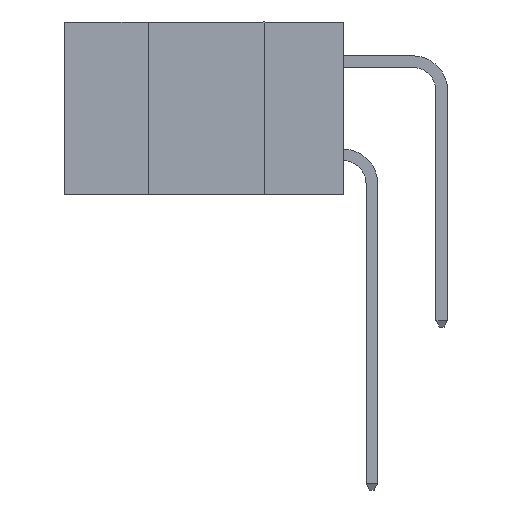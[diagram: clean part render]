
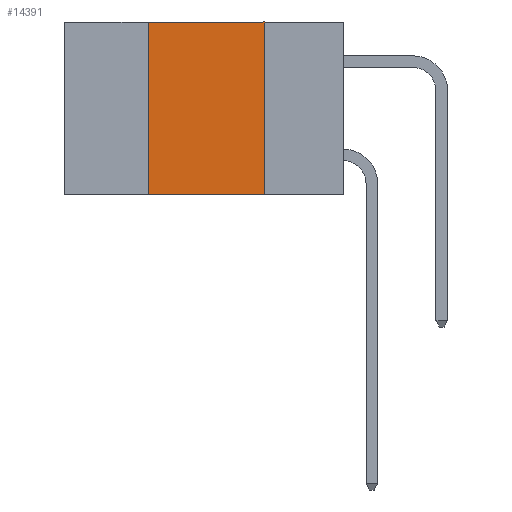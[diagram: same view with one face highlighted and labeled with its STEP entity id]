
A CAD part, left-side view. The second image highlights one B-rep face of the part: STEP entity #14391.
In plain terms, the highlighted planar face has unit normal (-1, 0, 0).
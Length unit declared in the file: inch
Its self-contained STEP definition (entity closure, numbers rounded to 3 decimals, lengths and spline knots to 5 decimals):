
#1706 = LINE ( 'NONE', #13991, #2848 ) ;
#2848 = VECTOR ( 'NONE', #13791, 39.37008 ) ;
#4884 = PLANE ( 'NONE',  #15498 ) ;
#5731 = VERTEX_POINT ( 'NONE', #10891 ) ;
#5781 = LINE ( 'NONE', #11690, #9344 ) ;
#6665 = DIRECTION ( 'NONE',  ( 0., 0., -1. ) ) ;
#6890 = CARTESIAN_POINT ( 'NONE',  ( 0., 0.17, -0.37 ) ) ;
#6941 = ORIENTED_EDGE ( 'NONE', *, *, #12278, .F. ) ;
#7290 = EDGE_LOOP ( 'NONE', ( #6941, #21047, #7484, #17150 ) ) ;
#7484 = ORIENTED_EDGE ( 'NONE', *, *, #7670, .F. ) ;
#7536 = CARTESIAN_POINT ( 'NONE',  ( 0., 0.42, 0. ) ) ;
#7670 = EDGE_CURVE ( 'NONE', #5731, #15430, #1706, .T. ) ;
#9344 = VECTOR ( 'NONE', #16772, 39.37008 ) ;
#9992 = EDGE_CURVE ( 'NONE', #5731, #14489, #5781, .T. ) ;
#10398 = DIRECTION ( 'NONE',  ( 0., 0., -1. ) ) ;
#10891 = CARTESIAN_POINT ( 'NONE',  ( 0., 0.42, -0.37 ) ) ;
#11690 = CARTESIAN_POINT ( 'NONE',  ( 0., 0.6, -0.37 ) ) ;
#11728 = FACE_OUTER_BOUND ( 'NONE', #7290, .T. ) ;
#12278 = EDGE_CURVE ( 'NONE', #13889, #14489, #14766, .T. ) ;
#12845 = VECTOR ( 'NONE', #16999, 39.37008 ) ;
#13424 = EDGE_CURVE ( 'NONE', #15430, #13889, #17380, .T. ) ;
#13566 = CARTESIAN_POINT ( 'NONE',  ( 0., 0.6, 0. ) ) ;
#13791 = DIRECTION ( 'NONE',  ( 0., 0., 1. ) ) ;
#13889 = VERTEX_POINT ( 'NONE', #16382 ) ;
#13991 = CARTESIAN_POINT ( 'NONE',  ( 0., 0.42, -0.37 ) ) ;
#14230 = VECTOR ( 'NONE', #10398, 39.37008 ) ;
#14391 = ADVANCED_FACE ( 'NONE', ( #11728 ), #4884, .F. ) ;
#14489 = VERTEX_POINT ( 'NONE', #6890 ) ;
#14766 = LINE ( 'NONE', #15480, #14230 ) ;
#15242 = CARTESIAN_POINT ( 'NONE',  ( 0., 0.6, 0. ) ) ;
#15430 = VERTEX_POINT ( 'NONE', #7536 ) ;
#15480 = CARTESIAN_POINT ( 'NONE',  ( 0., 0.17, -0.37 ) ) ;
#15498 = AXIS2_PLACEMENT_3D ( 'NONE', #15242, #16936, #6665 ) ;
#16382 = CARTESIAN_POINT ( 'NONE',  ( 0., 0.17, 0. ) ) ;
#16772 = DIRECTION ( 'NONE',  ( 0., -1., 0. ) ) ;
#16936 = DIRECTION ( 'NONE',  ( 1., 0., 0. ) ) ;
#16999 = DIRECTION ( 'NONE',  ( 0., -1., 0. ) ) ;
#17150 = ORIENTED_EDGE ( 'NONE', *, *, #9992, .T. ) ;
#17380 = LINE ( 'NONE', #13566, #12845 ) ;
#21047 = ORIENTED_EDGE ( 'NONE', *, *, #13424, .F. ) ;
